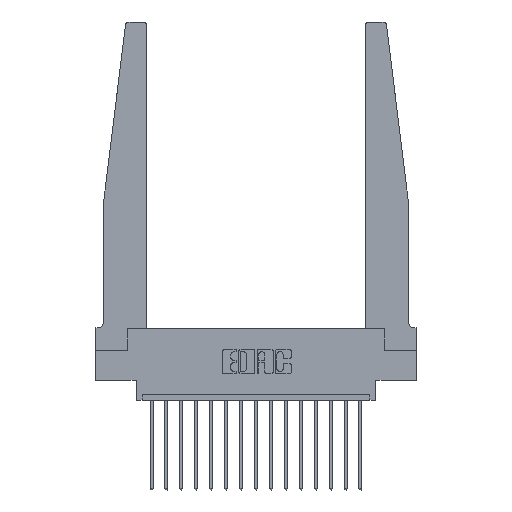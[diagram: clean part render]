
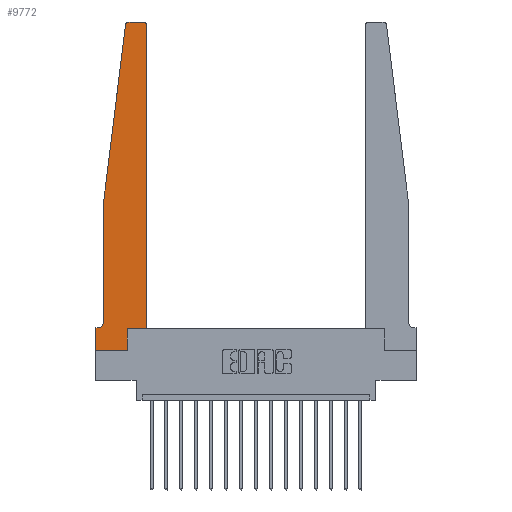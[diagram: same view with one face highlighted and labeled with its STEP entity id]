
A CAD part, top view. The second image highlights one B-rep face of the part: STEP entity #9772.
In plain terms, the highlighted planar face has unit normal (0, 0, 1).
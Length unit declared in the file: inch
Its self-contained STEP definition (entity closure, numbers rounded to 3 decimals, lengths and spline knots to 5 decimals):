
#200 = CARTESIAN_POINT ( 'NONE',  ( 0.395, 2.75, 0.37 ) ) ;
#325 = CARTESIAN_POINT ( 'NONE',  ( 0., 0.1875, 0.37 ) ) ;
#360 = CARTESIAN_POINT ( 'NONE',  ( 0.065, 1.25, 0.37 ) ) ;
#400 = EDGE_CURVE ( 'NONE', #14550, #6748, #1711, .T. ) ;
#469 = CARTESIAN_POINT ( 'NONE',  ( 0., 0.1875, 0.37 ) ) ;
#500 = ORIENTED_EDGE ( 'NONE', *, *, #13932, .T. ) ;
#576 = DIRECTION ( 'NONE',  ( 0., 0., -1. ) ) ;
#622 = DIRECTION ( 'NONE',  ( 1., 0., 0. ) ) ;
#714 = CARTESIAN_POINT ( 'NONE',  ( 0.065, 1.25, 0.37 ) ) ;
#826 = EDGE_CURVE ( 'NONE', #1111, #14170, #4480, .T. ) ;
#1008 = VERTEX_POINT ( 'NONE', #2167 ) ;
#1111 = VERTEX_POINT ( 'NONE', #3385 ) ;
#1238 = ORIENTED_EDGE ( 'NONE', *, *, #14678, .T. ) ;
#1711 = LINE ( 'NONE', #9997, #8365 ) ;
#1755 = DIRECTION ( 'NONE',  ( 0., -1., 0. ) ) ;
#2028 = LINE ( 'NONE', #16791, #7003 ) ;
#2051 = CARTESIAN_POINT ( 'NONE',  ( 0.425, 0.18, 0.37 ) ) ;
#2167 = CARTESIAN_POINT ( 'NONE',  ( 0.27653, 2.75, 0.37 ) ) ;
#2629 = EDGE_CURVE ( 'NONE', #8014, #5803, #9865, .T. ) ;
#2670 = ORIENTED_EDGE ( 'NONE', *, *, #826, .T. ) ;
#2732 = CARTESIAN_POINT ( 'NONE',  ( 0.425, 2.72, 0.37 ) ) ;
#3058 = CARTESIAN_POINT ( 'NONE',  ( 0.395, 2.72, 0.37 ) ) ;
#3150 = AXIS2_PLACEMENT_3D ( 'NONE', #14386, #17019, #622 ) ;
#3184 = ORIENTED_EDGE ( 'NONE', *, *, #2629, .T. ) ;
#3385 = CARTESIAN_POINT ( 'NONE',  ( 0.2605, 0.18, 0.37 ) ) ;
#3428 = VECTOR ( 'NONE', #8787, 39.37008 ) ;
#3861 = CARTESIAN_POINT ( 'NONE',  ( 0.065, 0.2375, 0.37 ) ) ;
#3925 = VERTEX_POINT ( 'NONE', #325 ) ;
#4371 = ORIENTED_EDGE ( 'NONE', *, *, #9832, .T. ) ;
#4460 = LINE ( 'NONE', #16070, #5986 ) ;
#4480 = LINE ( 'NONE', #8087, #16540 ) ;
#4607 = ORIENTED_EDGE ( 'NONE', *, *, #7400, .T. ) ;
#4744 = CARTESIAN_POINT ( 'NONE',  ( 0.425, 0.18, 0.37 ) ) ;
#4860 = VERTEX_POINT ( 'NONE', #3861 ) ;
#4940 = DIRECTION ( 'NONE',  ( 0., 0., 1. ) ) ;
#5009 = AXIS2_PLACEMENT_3D ( 'NONE', #469, #4940, #7587 ) ;
#5306 = AXIS2_PLACEMENT_3D ( 'NONE', #7516, #576, #7625 ) ;
#5485 = ORIENTED_EDGE ( 'NONE', *, *, #11166, .T. ) ;
#5758 = ORIENTED_EDGE ( 'NONE', *, *, #11215, .T. ) ;
#5803 = VERTEX_POINT ( 'NONE', #200 ) ;
#5986 = VECTOR ( 'NONE', #9164, 39.37008 ) ;
#6041 = LINE ( 'NONE', #4744, #3428 ) ;
#6128 = VECTOR ( 'NONE', #13174, 39.37008 ) ;
#6159 = PLANE ( 'NONE',  #5009 ) ;
#6212 = CARTESIAN_POINT ( 'NONE',  ( 0., 0., 0.37 ) ) ;
#6401 = ORIENTED_EDGE ( 'NONE', *, *, #14782, .T. ) ;
#6557 = VERTEX_POINT ( 'NONE', #14220 ) ;
#6743 = EDGE_CURVE ( 'NONE', #5803, #1008, #4460, .T. ) ;
#6748 = VERTEX_POINT ( 'NONE', #714 ) ;
#6818 = CARTESIAN_POINT ( 'NONE',  ( 0.065, 0.1875, 0.37 ) ) ;
#7003 = VECTOR ( 'NONE', #10036, 39.37008 ) ;
#7102 = VECTOR ( 'NONE', #1755, 39.37008 ) ;
#7400 = EDGE_CURVE ( 'NONE', #16435, #3925, #15441, .T. ) ;
#7516 = CARTESIAN_POINT ( 'NONE',  ( 0.015, 0.2375, 0.37 ) ) ;
#7580 = AXIS2_PLACEMENT_3D ( 'NONE', #3058, #10071, #12842 ) ;
#7587 = DIRECTION ( 'NONE',  ( 1., 0., 0. ) ) ;
#7625 = DIRECTION ( 'NONE',  ( -1., 0., 0. ) ) ;
#7641 = CARTESIAN_POINT ( 'NONE',  ( 0.2605, 0., 0.37 ) ) ;
#7675 = EDGE_CURVE ( 'NONE', #1008, #14550, #13942, .T. ) ;
#8014 = VERTEX_POINT ( 'NONE', #2732 ) ;
#8087 = CARTESIAN_POINT ( 'NONE',  ( 0.425, 0.18, 0.37 ) ) ;
#8224 = ORIENTED_EDGE ( 'NONE', *, *, #6743, .T. ) ;
#8365 = VECTOR ( 'NONE', #12822, 39.37008 ) ;
#8787 = DIRECTION ( 'NONE',  ( 0., 1., 0. ) ) ;
#9164 = DIRECTION ( 'NONE',  ( -1., 0., 0. ) ) ;
#9772 = ADVANCED_FACE ( 'NONE', ( #12160 ), #6159, .T. ) ;
#9784 = VERTEX_POINT ( 'NONE', #7641 ) ;
#9805 = LINE ( 'NONE', #6212, #6128 ) ;
#9832 = EDGE_CURVE ( 'NONE', #6557, #9784, #9805, .T. ) ;
#9865 = CIRCLE ( 'NONE', #7580, 0.03 ) ;
#9997 = CARTESIAN_POINT ( 'NONE',  ( 0.065, 1.25, 0.37 ) ) ;
#10036 = DIRECTION ( 'NONE',  ( 0., 1., 0. ) ) ;
#10071 = DIRECTION ( 'NONE',  ( 0., 0., 1. ) ) ;
#10998 = DIRECTION ( 'NONE',  ( -1., 0., 0. ) ) ;
#11166 = EDGE_CURVE ( 'NONE', #6748, #4860, #12296, .T. ) ;
#11215 = EDGE_CURVE ( 'NONE', #14170, #8014, #6041, .T. ) ;
#11799 = EDGE_LOOP ( 'NONE', ( #8224, #13383, #14489, #5485, #6401, #4607, #500, #4371, #1238, #2670, #5758, #3184 ) ) ;
#12081 = CARTESIAN_POINT ( 'NONE',  ( 0., 0., 0.37 ) ) ;
#12160 = FACE_OUTER_BOUND ( 'NONE', #11799, .T. ) ;
#12296 = LINE ( 'NONE', #360, #7102 ) ;
#12452 = DIRECTION ( 'NONE',  ( 1., 0., 0. ) ) ;
#12665 = VECTOR ( 'NONE', #10998, 39.37008 ) ;
#12822 = DIRECTION ( 'NONE',  ( -0.122, -0.992, 0. ) ) ;
#12842 = DIRECTION ( 'NONE',  ( 1., 0., 0. ) ) ;
#13174 = DIRECTION ( 'NONE',  ( 1., 0., 0. ) ) ;
#13383 = ORIENTED_EDGE ( 'NONE', *, *, #7675, .T. ) ;
#13932 = EDGE_CURVE ( 'NONE', #3925, #6557, #17788, .T. ) ;
#13942 = CIRCLE ( 'NONE', #3150, 0.03 ) ;
#14170 = VERTEX_POINT ( 'NONE', #2051 ) ;
#14220 = CARTESIAN_POINT ( 'NONE',  ( 0., 0., 0.37 ) ) ;
#14337 = CARTESIAN_POINT ( 'NONE',  ( 0.015, 0.1875, 0.37 ) ) ;
#14386 = CARTESIAN_POINT ( 'NONE',  ( 0.27653, 2.72, 0.37 ) ) ;
#14489 = ORIENTED_EDGE ( 'NONE', *, *, #400, .T. ) ;
#14550 = VERTEX_POINT ( 'NONE', #15112 ) ;
#14678 = EDGE_CURVE ( 'NONE', #9784, #1111, #2028, .T. ) ;
#14782 = EDGE_CURVE ( 'NONE', #4860, #16435, #17336, .T. ) ;
#15112 = CARTESIAN_POINT ( 'NONE',  ( 0.24675, 2.72367, 0.37 ) ) ;
#15441 = LINE ( 'NONE', #6818, #12665 ) ;
#16070 = CARTESIAN_POINT ( 'NONE',  ( 0.25, 2.75, 0.37 ) ) ;
#16219 = DIRECTION ( 'NONE',  ( 0., -1., 0. ) ) ;
#16435 = VERTEX_POINT ( 'NONE', #14337 ) ;
#16480 = VECTOR ( 'NONE', #16219, 39.37008 ) ;
#16540 = VECTOR ( 'NONE', #12452, 39.37008 ) ;
#16791 = CARTESIAN_POINT ( 'NONE',  ( 0.2605, 0.18, 0.37 ) ) ;
#17019 = DIRECTION ( 'NONE',  ( 0., 0., 1. ) ) ;
#17336 = CIRCLE ( 'NONE', #5306, 0.05 ) ;
#17788 = LINE ( 'NONE', #12081, #16480 ) ;
